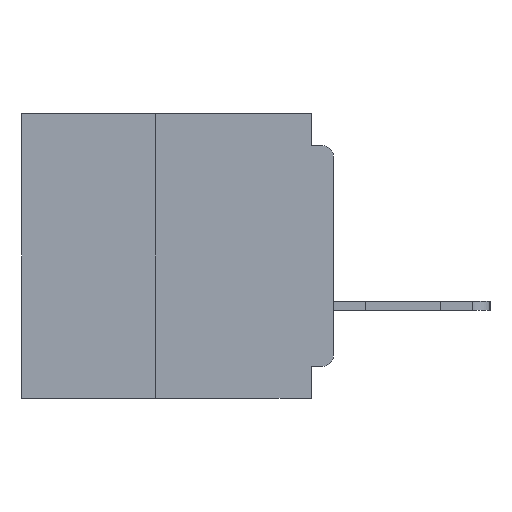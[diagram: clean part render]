
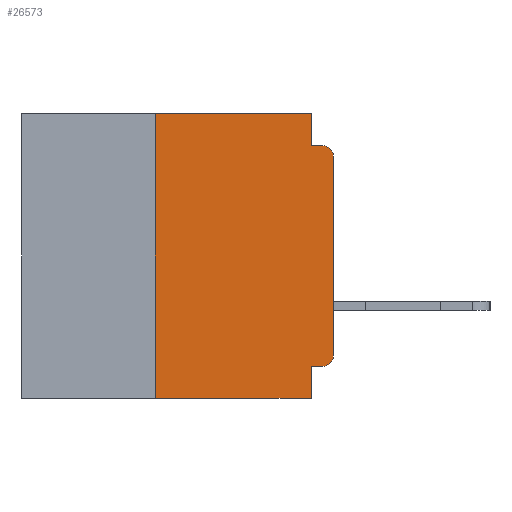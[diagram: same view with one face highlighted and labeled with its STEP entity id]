
A CAD part, left-side view. The second image highlights one B-rep face of the part: STEP entity #26573.
In plain terms, the highlighted planar face has unit normal (-1, 0, 0).
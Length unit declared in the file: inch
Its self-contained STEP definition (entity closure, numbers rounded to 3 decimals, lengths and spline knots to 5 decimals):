
#477 = ORIENTED_EDGE ( 'NONE', *, *, #35810, .F. ) ;
#1356 = VECTOR ( 'NONE', #25313, 39.37008 ) ;
#2071 = VERTEX_POINT ( 'NONE', #39651 ) ;
#2284 = CARTESIAN_POINT ( 'NONE',  ( 0., 0., -0.06 ) ) ;
#2446 = ORIENTED_EDGE ( 'NONE', *, *, #22289, .T. ) ;
#2666 = AXIS2_PLACEMENT_3D ( 'NONE', #15463, #37160, #18625 ) ;
#3939 = LINE ( 'NONE', #35734, #19577 ) ;
#4447 = LINE ( 'NONE', #24278, #20088 ) ;
#4601 = VECTOR ( 'NONE', #13031, 39.37008 ) ;
#5075 = ORIENTED_EDGE ( 'NONE', *, *, #33451, .F. ) ;
#5548 = EDGE_CURVE ( 'NONE', #6482, #31347, #27098, .T. ) ;
#5964 = VECTOR ( 'NONE', #10135, 39.37008 ) ;
#6316 = CARTESIAN_POINT ( 'NONE',  ( 0., 0.437, -0.4 ) ) ;
#6482 = VERTEX_POINT ( 'NONE', #15007 ) ;
#6629 = CARTESIAN_POINT ( 'NONE',  ( 0., 0., -0.355 ) ) ;
#6778 = DIRECTION ( 'NONE',  ( -1., 0., 0. ) ) ;
#6899 = DIRECTION ( 'NONE',  ( 1., 0., 0. ) ) ;
#7315 = DIRECTION ( 'NONE',  ( 0., 0., -1. ) ) ;
#7572 = CARTESIAN_POINT ( 'NONE',  ( 0., 0.031, -0.355 ) ) ;
#8093 = CARTESIAN_POINT ( 'NONE',  ( 0., 0., -0.34 ) ) ;
#8534 = LINE ( 'NONE', #26024, #32454 ) ;
#9386 = ORIENTED_EDGE ( 'NONE', *, *, #18080, .F. ) ;
#9405 = DIRECTION ( 'NONE',  ( 0., -1., 0. ) ) ;
#9848 = CARTESIAN_POINT ( 'NONE',  ( 0., 0., -0.045 ) ) ;
#10135 = DIRECTION ( 'NONE',  ( 0., 0., -1. ) ) ;
#11072 = CARTESIAN_POINT ( 'NONE',  ( 0., 0.031, 0. ) ) ;
#11816 = VERTEX_POINT ( 'NONE', #2284 ) ;
#11905 = AXIS2_PLACEMENT_3D ( 'NONE', #34656, #6899, #28763 ) ;
#12919 = VERTEX_POINT ( 'NONE', #35768 ) ;
#13031 = DIRECTION ( 'NONE',  ( 0., -1., 0. ) ) ;
#13098 = EDGE_CURVE ( 'NONE', #34182, #15677, #4447, .T. ) ;
#13786 = ORIENTED_EDGE ( 'NONE', *, *, #17880, .T. ) ;
#14022 = DIRECTION ( 'NONE',  ( 0., 0., 1. ) ) ;
#14031 = EDGE_LOOP ( 'NONE', ( #35464, #13786, #40220, #22479, #32939, #9386, #17910, #5075, #477, #2446 ) ) ;
#14897 = EDGE_CURVE ( 'NONE', #15677, #12919, #8534, .T. ) ;
#15007 = CARTESIAN_POINT ( 'NONE',  ( 0., 0.25, -0.4 ) ) ;
#15422 = EDGE_CURVE ( 'NONE', #12919, #2071, #29502, .T. ) ;
#15463 = CARTESIAN_POINT ( 'NONE',  ( 0., 0.015, -0.34 ) ) ;
#15677 = VERTEX_POINT ( 'NONE', #11072 ) ;
#17563 = CARTESIAN_POINT ( 'NONE',  ( 0., 0.031, -0.4 ) ) ;
#17880 = EDGE_CURVE ( 'NONE', #11816, #2071, #19522, .T. ) ;
#17910 = ORIENTED_EDGE ( 'NONE', *, *, #5548, .T. ) ;
#18080 = EDGE_CURVE ( 'NONE', #6482, #34182, #3939, .T. ) ;
#18625 = DIRECTION ( 'NONE',  ( 0., 0., -1. ) ) ;
#18807 = VECTOR ( 'NONE', #9405, 39.37008 ) ;
#19341 = PLANE ( 'NONE',  #11905 ) ;
#19522 = CIRCLE ( 'NONE', #24979, 0.015 ) ;
#19577 = VECTOR ( 'NONE', #14022, 39.37008 ) ;
#20088 = VECTOR ( 'NONE', #27420, 39.37008 ) ;
#21235 = CIRCLE ( 'NONE', #2666, 0.015 ) ;
#22289 = EDGE_CURVE ( 'NONE', #27851, #24098, #21235, .T. ) ;
#22479 = ORIENTED_EDGE ( 'NONE', *, *, #14897, .F. ) ;
#24098 = VERTEX_POINT ( 'NONE', #8093 ) ;
#24188 = CARTESIAN_POINT ( 'NONE',  ( 0., 0., 0. ) ) ;
#24278 = CARTESIAN_POINT ( 'NONE',  ( 0., 0.437, 0. ) ) ;
#24979 = AXIS2_PLACEMENT_3D ( 'NONE', #25477, #6778, #28638 ) ;
#25313 = DIRECTION ( 'NONE',  ( 0., 1., 0. ) ) ;
#25477 = CARTESIAN_POINT ( 'NONE',  ( 0., 0.015, -0.06 ) ) ;
#26024 = CARTESIAN_POINT ( 'NONE',  ( 0., 0.031, 0. ) ) ;
#26573 = ADVANCED_FACE ( 'NONE', ( #33809 ), #19341, .F. ) ;
#27098 = LINE ( 'NONE', #6316, #18807 ) ;
#27309 = DIRECTION ( 'NONE',  ( 0., 0., 1. ) ) ;
#27420 = DIRECTION ( 'NONE',  ( 0., -1., 0. ) ) ;
#27851 = VERTEX_POINT ( 'NONE', #35505 ) ;
#28638 = DIRECTION ( 'NONE',  ( 0., 0., -1. ) ) ;
#28763 = DIRECTION ( 'NONE',  ( 0., 0., -1. ) ) ;
#29502 = LINE ( 'NONE', #9848, #4601 ) ;
#30623 = EDGE_CURVE ( 'NONE', #24098, #11816, #39653, .T. ) ;
#30869 = LINE ( 'NONE', #31993, #5964 ) ;
#31347 = VERTEX_POINT ( 'NONE', #17563 ) ;
#31993 = CARTESIAN_POINT ( 'NONE',  ( 0., 0.031, -0.4 ) ) ;
#32454 = VECTOR ( 'NONE', #7315, 39.37008 ) ;
#32939 = ORIENTED_EDGE ( 'NONE', *, *, #13098, .F. ) ;
#33451 = EDGE_CURVE ( 'NONE', #34109, #31347, #30869, .T. ) ;
#33809 = FACE_OUTER_BOUND ( 'NONE', #14031, .T. ) ;
#34109 = VERTEX_POINT ( 'NONE', #7572 ) ;
#34182 = VERTEX_POINT ( 'NONE', #38896 ) ;
#34656 = CARTESIAN_POINT ( 'NONE',  ( 0., 0.437, 0. ) ) ;
#35414 = LINE ( 'NONE', #6629, #1356 ) ;
#35464 = ORIENTED_EDGE ( 'NONE', *, *, #30623, .T. ) ;
#35505 = CARTESIAN_POINT ( 'NONE',  ( 0., 0.015, -0.355 ) ) ;
#35734 = CARTESIAN_POINT ( 'NONE',  ( 0., 0.25, -0.4 ) ) ;
#35768 = CARTESIAN_POINT ( 'NONE',  ( 0., 0.031, -0.045 ) ) ;
#35810 = EDGE_CURVE ( 'NONE', #27851, #34109, #35414, .T. ) ;
#37160 = DIRECTION ( 'NONE',  ( -1., 0., 0. ) ) ;
#37727 = VECTOR ( 'NONE', #27309, 39.37008 ) ;
#38896 = CARTESIAN_POINT ( 'NONE',  ( 0., 0.25, 0. ) ) ;
#39651 = CARTESIAN_POINT ( 'NONE',  ( 0., 0.015, -0.045 ) ) ;
#39653 = LINE ( 'NONE', #24188, #37727 ) ;
#40220 = ORIENTED_EDGE ( 'NONE', *, *, #15422, .F. ) ;
